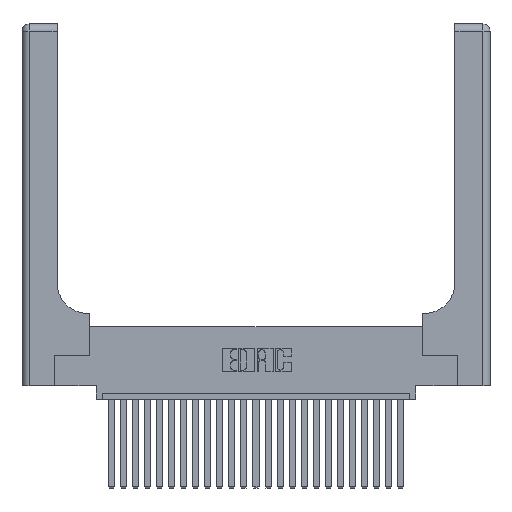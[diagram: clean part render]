
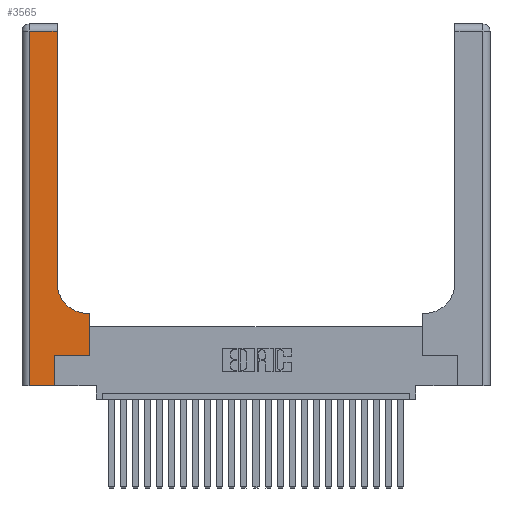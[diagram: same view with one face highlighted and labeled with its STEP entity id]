
A CAD part, top view. The second image highlights one B-rep face of the part: STEP entity #3565.
In plain terms, the highlighted planar face has unit normal (0, 0, 1).
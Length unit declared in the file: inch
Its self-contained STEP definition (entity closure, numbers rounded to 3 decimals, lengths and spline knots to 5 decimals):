
#336 = VECTOR ( 'NONE', #23037, 39.37008 ) ;
#350 = ORIENTED_EDGE ( 'NONE', *, *, #8407, .T. ) ;
#404 = CIRCLE ( 'NONE', #24664, 0.25 ) ;
#487 = CARTESIAN_POINT ( 'NONE',  ( 0.2915, 2.94, 0.37 ) ) ;
#1470 = DIRECTION ( 'NONE',  ( 1., 0., 0. ) ) ;
#1689 = VERTEX_POINT ( 'NONE', #487 ) ;
#1992 = DIRECTION ( 'NONE',  ( 0., 1., 0. ) ) ;
#2443 = ORIENTED_EDGE ( 'NONE', *, *, #25284, .T. ) ;
#2684 = ORIENTED_EDGE ( 'NONE', *, *, #4315, .T. ) ;
#3355 = CARTESIAN_POINT ( 'NONE',  ( 0.5585, 0.25, 0.37 ) ) ;
#3465 = CARTESIAN_POINT ( 'NONE',  ( 0.2915, 3., 0.37 ) ) ;
#3565 = ADVANCED_FACE ( 'NONE', ( #25549 ), #10101, .F. ) ;
#3998 = VECTOR ( 'NONE', #12781, 39.37008 ) ;
#4315 = EDGE_CURVE ( 'NONE', #25087, #15981, #17608, .T. ) ;
#4568 = CARTESIAN_POINT ( 'NONE',  ( 0.5415, 0.85, 0.37 ) ) ;
#5850 = DIRECTION ( 'NONE',  ( -1., 0., 0. ) ) ;
#6004 = VECTOR ( 'NONE', #1470, 39.37008 ) ;
#6184 = CARTESIAN_POINT ( 'NONE',  ( 0.269, 0., 0.37 ) ) ;
#6815 = VERTEX_POINT ( 'NONE', #23705 ) ;
#7627 = CARTESIAN_POINT ( 'NONE',  ( 0.269, 0.25, 0.37 ) ) ;
#8325 = DIRECTION ( 'NONE',  ( 0., 1., 0. ) ) ;
#8407 = EDGE_CURVE ( 'NONE', #15981, #9214, #404, .T. ) ;
#8834 = LINE ( 'NONE', #3465, #20173 ) ;
#8946 = DIRECTION ( 'NONE',  ( 1., 0., 0. ) ) ;
#9214 = VERTEX_POINT ( 'NONE', #10142 ) ;
#9832 = VERTEX_POINT ( 'NONE', #12583 ) ;
#10101 = PLANE ( 'NONE',  #24090 ) ;
#10142 = CARTESIAN_POINT ( 'NONE',  ( 0.2915, 0.85, 0.37 ) ) ;
#10854 = ORIENTED_EDGE ( 'NONE', *, *, #13436, .T. ) ;
#11386 = LINE ( 'NONE', #7627, #6004 ) ;
#11616 = VECTOR ( 'NONE', #25972, 39.37008 ) ;
#12450 = CARTESIAN_POINT ( 'NONE',  ( 0.5585, 0.25, 0.37 ) ) ;
#12583 = CARTESIAN_POINT ( 'NONE',  ( 0.269, 0., 0.37 ) ) ;
#12781 = DIRECTION ( 'NONE',  ( 1., 0., 0. ) ) ;
#13293 = DIRECTION ( 'NONE',  ( 0., 1., 0. ) ) ;
#13350 = ORIENTED_EDGE ( 'NONE', *, *, #26206, .T. ) ;
#13419 = VECTOR ( 'NONE', #1992, 39.37008 ) ;
#13436 = EDGE_CURVE ( 'NONE', #1689, #23557, #21055, .T. ) ;
#14605 = ORIENTED_EDGE ( 'NONE', *, *, #23660, .T. ) ;
#14726 = LINE ( 'NONE', #19019, #3998 ) ;
#14973 = LINE ( 'NONE', #6184, #13419 ) ;
#14992 = CARTESIAN_POINT ( 'NONE',  ( 0.06, 3., 0.37 ) ) ;
#15809 = CARTESIAN_POINT ( 'NONE',  ( 0., 3., 0.37 ) ) ;
#15981 = VERTEX_POINT ( 'NONE', #22811 ) ;
#16115 = ORIENTED_EDGE ( 'NONE', *, *, #21507, .T. ) ;
#16171 = DIRECTION ( 'NONE',  ( 0., 0., -1. ) ) ;
#16352 = CARTESIAN_POINT ( 'NONE',  ( 0., 2.94, 0.37 ) ) ;
#17044 = CARTESIAN_POINT ( 'NONE',  ( 0.269, 0.25, 0.37 ) ) ;
#17455 = LINE ( 'NONE', #14992, #336 ) ;
#17608 = LINE ( 'NONE', #19779, #11616 ) ;
#17987 = CARTESIAN_POINT ( 'NONE',  ( 0.5585, 0.6, 0.37 ) ) ;
#19019 = CARTESIAN_POINT ( 'NONE',  ( 0., 0., 0.37 ) ) ;
#19069 = VERTEX_POINT ( 'NONE', #17044 ) ;
#19086 = LINE ( 'NONE', #12450, #20349 ) ;
#19779 = CARTESIAN_POINT ( 'NONE',  ( 0.2915, 0.6, 0.37 ) ) ;
#19989 = ORIENTED_EDGE ( 'NONE', *, *, #22959, .T. ) ;
#20173 = VECTOR ( 'NONE', #13293, 39.37008 ) ;
#20349 = VECTOR ( 'NONE', #8325, 39.37008 ) ;
#20671 = DIRECTION ( 'NONE',  ( -1., 0., 0. ) ) ;
#21055 = LINE ( 'NONE', #16352, #23594 ) ;
#21507 = EDGE_CURVE ( 'NONE', #23557, #6815, #17455, .T. ) ;
#22593 = EDGE_LOOP ( 'NONE', ( #14605, #10854, #16115, #2443, #25029, #19989, #13350, #2684, #350 ) ) ;
#22811 = CARTESIAN_POINT ( 'NONE',  ( 0.5415, 0.6, 0.37 ) ) ;
#22836 = VERTEX_POINT ( 'NONE', #3355 ) ;
#22959 = EDGE_CURVE ( 'NONE', #19069, #22836, #11386, .T. ) ;
#23037 = DIRECTION ( 'NONE',  ( 0., -1., 0. ) ) ;
#23557 = VERTEX_POINT ( 'NONE', #25225 ) ;
#23594 = VECTOR ( 'NONE', #20671, 39.37008 ) ;
#23660 = EDGE_CURVE ( 'NONE', #9214, #1689, #8834, .T. ) ;
#23705 = CARTESIAN_POINT ( 'NONE',  ( 0.06, 0., 0.37 ) ) ;
#23943 = DIRECTION ( 'NONE',  ( 0., 0., -1. ) ) ;
#24090 = AXIS2_PLACEMENT_3D ( 'NONE', #15809, #23943, #5850 ) ;
#24664 = AXIS2_PLACEMENT_3D ( 'NONE', #4568, #16171, #8946 ) ;
#25029 = ORIENTED_EDGE ( 'NONE', *, *, #26227, .T. ) ;
#25087 = VERTEX_POINT ( 'NONE', #17987 ) ;
#25225 = CARTESIAN_POINT ( 'NONE',  ( 0.06, 2.94, 0.37 ) ) ;
#25284 = EDGE_CURVE ( 'NONE', #6815, #9832, #14726, .T. ) ;
#25549 = FACE_OUTER_BOUND ( 'NONE', #22593, .T. ) ;
#25972 = DIRECTION ( 'NONE',  ( -1., 0., 0. ) ) ;
#26206 = EDGE_CURVE ( 'NONE', #22836, #25087, #19086, .T. ) ;
#26227 = EDGE_CURVE ( 'NONE', #9832, #19069, #14973, .T. ) ;
